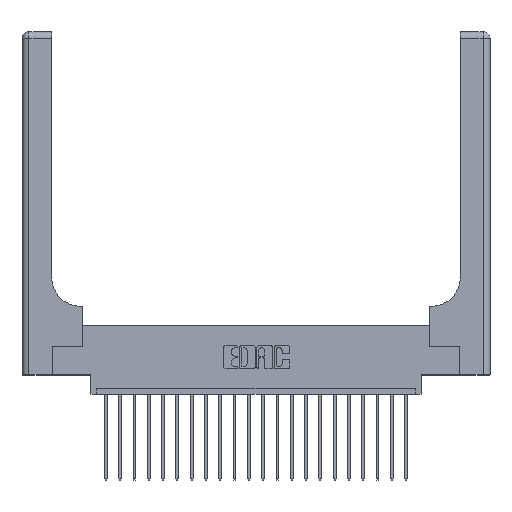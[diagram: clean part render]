
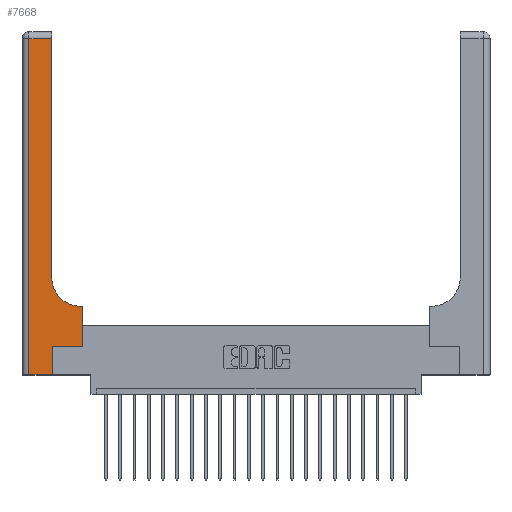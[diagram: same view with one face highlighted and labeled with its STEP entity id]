
A CAD part, top view. The second image highlights one B-rep face of the part: STEP entity #7668.
In plain terms, the highlighted planar face has unit normal (0, 0, 1).
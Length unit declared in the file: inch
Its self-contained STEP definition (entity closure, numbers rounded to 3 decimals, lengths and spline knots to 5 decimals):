
#504 = DIRECTION ( 'NONE',  ( 0., 0., -1. ) ) ;
#723 = VERTEX_POINT ( 'NONE', #11329 ) ;
#885 = EDGE_CURVE ( 'NONE', #11598, #12424, #21291, .T. ) ;
#1337 = CARTESIAN_POINT ( 'NONE',  ( 0.26, 3., 0.37 ) ) ;
#1364 = VECTOR ( 'NONE', #7762, 39.37008 ) ;
#1449 = CARTESIAN_POINT ( 'NONE',  ( 0., 3., 0.37 ) ) ;
#1550 = ORIENTED_EDGE ( 'NONE', *, *, #21560, .T. ) ;
#1720 = EDGE_CURVE ( 'NONE', #723, #19400, #11376, .T. ) ;
#2169 = VERTEX_POINT ( 'NONE', #11351 ) ;
#2250 = DIRECTION ( 'NONE',  ( -1., 0., 0. ) ) ;
#2718 = LINE ( 'NONE', #4632, #4555 ) ;
#3774 = VECTOR ( 'NONE', #13458, 39.37008 ) ;
#3799 = CARTESIAN_POINT ( 'NONE',  ( 0.26, 2.94, 0.37 ) ) ;
#3884 = VECTOR ( 'NONE', #16159, 39.37008 ) ;
#4144 = EDGE_LOOP ( 'NONE', ( #18778, #20104, #8656, #21509, #15515, #8948, #4399, #15474, #1550 ) ) ;
#4399 = ORIENTED_EDGE ( 'NONE', *, *, #885, .T. ) ;
#4423 = EDGE_CURVE ( 'NONE', #21270, #2169, #5461, .T. ) ;
#4555 = VECTOR ( 'NONE', #13096, 39.37008 ) ;
#4632 = CARTESIAN_POINT ( 'NONE',  ( 0., 0., 0.37 ) ) ;
#4681 = VECTOR ( 'NONE', #4693, 39.37008 ) ;
#4693 = DIRECTION ( 'NONE',  ( 0., 1., 0. ) ) ;
#4757 = LINE ( 'NONE', #6850, #3774 ) ;
#5171 = CARTESIAN_POINT ( 'NONE',  ( 0.528, 0.25, 0.37 ) ) ;
#5246 = CARTESIAN_POINT ( 'NONE',  ( 0.06, 3., 0.37 ) ) ;
#5440 = VERTEX_POINT ( 'NONE', #19156 ) ;
#5461 = LINE ( 'NONE', #5246, #17583 ) ;
#5663 = DIRECTION ( 'NONE',  ( 1., 0., 0. ) ) ;
#5905 = AXIS2_PLACEMENT_3D ( 'NONE', #1449, #13284, #21684 ) ;
#6104 = DIRECTION ( 'NONE',  ( -1., 0., 0. ) ) ;
#6416 = EDGE_CURVE ( 'NONE', #19400, #21270, #12910, .T. ) ;
#6850 = CARTESIAN_POINT ( 'NONE',  ( 0.265, 0.25, 0.37 ) ) ;
#7668 = ADVANCED_FACE ( 'NONE', ( #9815 ), #13175, .F. ) ;
#7762 = DIRECTION ( 'NONE',  ( 0., 1., 0. ) ) ;
#7909 = VERTEX_POINT ( 'NONE', #18038 ) ;
#8070 = EDGE_CURVE ( 'NONE', #5440, #11598, #4757, .T. ) ;
#8656 = ORIENTED_EDGE ( 'NONE', *, *, #4423, .T. ) ;
#8948 = ORIENTED_EDGE ( 'NONE', *, *, #8070, .T. ) ;
#9329 = CIRCLE ( 'NONE', #17548, 0.25 ) ;
#9437 = CARTESIAN_POINT ( 'NONE',  ( 0.265, 0., 0.37 ) ) ;
#9815 = FACE_OUTER_BOUND ( 'NONE', #4144, .T. ) ;
#11227 = LINE ( 'NONE', #9437, #1364 ) ;
#11329 = CARTESIAN_POINT ( 'NONE',  ( 0.26, 0.85, 0.37 ) ) ;
#11351 = CARTESIAN_POINT ( 'NONE',  ( 0.06, 0., 0.37 ) ) ;
#11376 = LINE ( 'NONE', #1337, #4681 ) ;
#11489 = EDGE_CURVE ( 'NONE', #2169, #7909, #2718, .T. ) ;
#11598 = VERTEX_POINT ( 'NONE', #5171 ) ;
#11917 = VERTEX_POINT ( 'NONE', #20458 ) ;
#12270 = VECTOR ( 'NONE', #6104, 39.37008 ) ;
#12424 = VERTEX_POINT ( 'NONE', #14030 ) ;
#12606 = EDGE_CURVE ( 'NONE', #7909, #5440, #11227, .T. ) ;
#12910 = LINE ( 'NONE', #16396, #12270 ) ;
#13096 = DIRECTION ( 'NONE',  ( 1., 0., 0. ) ) ;
#13175 = PLANE ( 'NONE',  #5905 ) ;
#13284 = DIRECTION ( 'NONE',  ( 0., 0., -1. ) ) ;
#13458 = DIRECTION ( 'NONE',  ( 1., 0., 0. ) ) ;
#13766 = LINE ( 'NONE', #17458, #15729 ) ;
#14030 = CARTESIAN_POINT ( 'NONE',  ( 0.528, 0.6, 0.37 ) ) ;
#15474 = ORIENTED_EDGE ( 'NONE', *, *, #20407, .T. ) ;
#15515 = ORIENTED_EDGE ( 'NONE', *, *, #12606, .T. ) ;
#15729 = VECTOR ( 'NONE', #2250, 39.37008 ) ;
#16159 = DIRECTION ( 'NONE',  ( 0., 1., 0. ) ) ;
#16396 = CARTESIAN_POINT ( 'NONE',  ( 0., 2.94, 0.37 ) ) ;
#17458 = CARTESIAN_POINT ( 'NONE',  ( 0.26, 0.6, 0.37 ) ) ;
#17548 = AXIS2_PLACEMENT_3D ( 'NONE', #21172, #504, #5663 ) ;
#17583 = VECTOR ( 'NONE', #18663, 39.37008 ) ;
#18038 = CARTESIAN_POINT ( 'NONE',  ( 0.265, 0., 0.37 ) ) ;
#18663 = DIRECTION ( 'NONE',  ( 0., -1., 0. ) ) ;
#18778 = ORIENTED_EDGE ( 'NONE', *, *, #1720, .T. ) ;
#19156 = CARTESIAN_POINT ( 'NONE',  ( 0.265, 0.25, 0.37 ) ) ;
#19400 = VERTEX_POINT ( 'NONE', #3799 ) ;
#19414 = CARTESIAN_POINT ( 'NONE',  ( 0.06, 2.94, 0.37 ) ) ;
#20104 = ORIENTED_EDGE ( 'NONE', *, *, #6416, .T. ) ;
#20407 = EDGE_CURVE ( 'NONE', #12424, #11917, #13766, .T. ) ;
#20458 = CARTESIAN_POINT ( 'NONE',  ( 0.51, 0.6, 0.37 ) ) ;
#21172 = CARTESIAN_POINT ( 'NONE',  ( 0.51, 0.85, 0.37 ) ) ;
#21270 = VERTEX_POINT ( 'NONE', #19414 ) ;
#21291 = LINE ( 'NONE', #21753, #3884 ) ;
#21509 = ORIENTED_EDGE ( 'NONE', *, *, #11489, .T. ) ;
#21560 = EDGE_CURVE ( 'NONE', #11917, #723, #9329, .T. ) ;
#21684 = DIRECTION ( 'NONE',  ( -1., 0., 0. ) ) ;
#21753 = CARTESIAN_POINT ( 'NONE',  ( 0.528, 0.25, 0.37 ) ) ;
